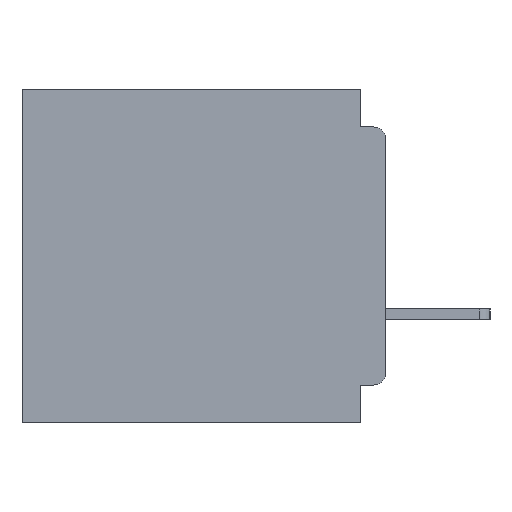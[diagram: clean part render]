
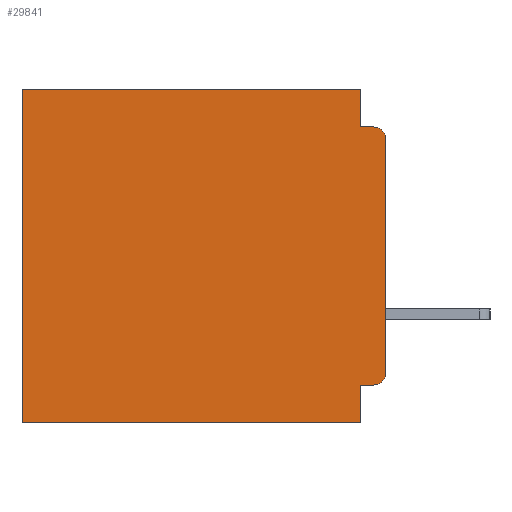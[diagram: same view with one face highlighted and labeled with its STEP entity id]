
A CAD part, left-side view. The second image highlights one B-rep face of the part: STEP entity #29841.
In plain terms, the highlighted planar face has unit normal (-1, 0, 0).
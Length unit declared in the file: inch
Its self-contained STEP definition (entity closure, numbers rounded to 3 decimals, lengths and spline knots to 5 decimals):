
#265 = VECTOR ( 'NONE', #46456, 39.37008 ) ;
#1572 = CARTESIAN_POINT ( 'NONE',  ( 0.3, 0.437, -0.4 ) ) ;
#1615 = EDGE_CURVE ( 'NONE', #7295, #20753, #33147, .T. ) ;
#2428 = LINE ( 'NONE', #33647, #3694 ) ;
#3460 = DIRECTION ( 'NONE',  ( 0., 1., 0. ) ) ;
#3662 = ORIENTED_EDGE ( 'NONE', *, *, #21971, .F. ) ;
#3694 = VECTOR ( 'NONE', #29589, 39.37008 ) ;
#4577 = DIRECTION ( 'NONE',  ( 1., 0., 0. ) ) ;
#5050 = VECTOR ( 'NONE', #21199, 39.37008 ) ;
#5406 = ORIENTED_EDGE ( 'NONE', *, *, #15258, .F. ) ;
#6187 = CARTESIAN_POINT ( 'NONE',  ( 0.3, 0.437, -0.4 ) ) ;
#6273 = ORIENTED_EDGE ( 'NONE', *, *, #46538, .F. ) ;
#6849 = EDGE_LOOP ( 'NONE', ( #51525, #38840, #45216, #6273, #16762, #49457, #3662, #35988, #5406, #42361 ) ) ;
#7295 = VERTEX_POINT ( 'NONE', #41009 ) ;
#7909 = DIRECTION ( 'NONE',  ( 0., 0., -1. ) ) ;
#9643 = VERTEX_POINT ( 'NONE', #45570 ) ;
#10082 = FACE_OUTER_BOUND ( 'NONE', #6849, .T. ) ;
#11104 = LINE ( 'NONE', #22349, #265 ) ;
#12404 = DIRECTION ( 'NONE',  ( 0., 0., -1. ) ) ;
#12607 = VECTOR ( 'NONE', #42141, 39.37008 ) ;
#12839 = VERTEX_POINT ( 'NONE', #47548 ) ;
#12994 = DIRECTION ( 'NONE',  ( -1., 0., 0. ) ) ;
#13832 = CARTESIAN_POINT ( 'NONE',  ( 0.3, 0., -0.4 ) ) ;
#13979 = VECTOR ( 'NONE', #3460, 39.37008 ) ;
#14029 = CARTESIAN_POINT ( 'NONE',  ( 0.3, 0., -0.34 ) ) ;
#15181 = LINE ( 'NONE', #13832, #12607 ) ;
#15258 = EDGE_CURVE ( 'NONE', #12839, #15596, #26531, .T. ) ;
#15596 = VERTEX_POINT ( 'NONE', #51578 ) ;
#16175 = CARTESIAN_POINT ( 'NONE',  ( 0.3, 0.031, -0.4 ) ) ;
#16762 = ORIENTED_EDGE ( 'NONE', *, *, #36141, .T. ) ;
#17529 = VECTOR ( 'NONE', #33875, 39.37008 ) ;
#17817 = CARTESIAN_POINT ( 'NONE',  ( 0.3, 0.015, -0.045 ) ) ;
#18796 = LINE ( 'NONE', #1572, #17529 ) ;
#19646 = EDGE_CURVE ( 'NONE', #7295, #28310, #43110, .T. ) ;
#20168 = VERTEX_POINT ( 'NONE', #46203 ) ;
#20345 = DIRECTION ( 'NONE',  ( -1., 0., 0. ) ) ;
#20721 = PLANE ( 'NONE',  #50280 ) ;
#20753 = VERTEX_POINT ( 'NONE', #17817 ) ;
#21199 = DIRECTION ( 'NONE',  ( 0., 1., 0. ) ) ;
#21971 = EDGE_CURVE ( 'NONE', #9643, #38137, #15181, .T. ) ;
#22255 = CARTESIAN_POINT ( 'NONE',  ( 0.3, 0.031, -0.045 ) ) ;
#22349 = CARTESIAN_POINT ( 'NONE',  ( 0.3, 0.031, 0. ) ) ;
#24540 = CARTESIAN_POINT ( 'NONE',  ( 0.3, 0., -0.4 ) ) ;
#26531 = LINE ( 'NONE', #49341, #5050 ) ;
#27902 = DIRECTION ( 'NONE',  ( 0., 0., -1. ) ) ;
#28310 = VERTEX_POINT ( 'NONE', #14029 ) ;
#28698 = CARTESIAN_POINT ( 'NONE',  ( 0.3, 0.015, -0.06 ) ) ;
#29589 = DIRECTION ( 'NONE',  ( 0., -1., 0. ) ) ;
#29841 = ADVANCED_FACE ( 'NONE', ( #10082 ), #20721, .F. ) ;
#29966 = AXIS2_PLACEMENT_3D ( 'NONE', #28698, #12994, #7909 ) ;
#32352 = VECTOR ( 'NONE', #12404, 39.37008 ) ;
#32781 = DIRECTION ( 'NONE',  ( 0., 0., -1. ) ) ;
#32958 = EDGE_CURVE ( 'NONE', #15596, #9643, #45087, .T. ) ;
#33018 = AXIS2_PLACEMENT_3D ( 'NONE', #44422, #20345, #48496 ) ;
#33069 = VECTOR ( 'NONE', #27902, 39.37008 ) ;
#33147 = CIRCLE ( 'NONE', #29966, 0.015 ) ;
#33647 = CARTESIAN_POINT ( 'NONE',  ( 0.3, 0., -0.045 ) ) ;
#33875 = DIRECTION ( 'NONE',  ( 0., 0., -1. ) ) ;
#34208 = VERTEX_POINT ( 'NONE', #22255 ) ;
#35339 = LINE ( 'NONE', #47908, #13979 ) ;
#35988 = ORIENTED_EDGE ( 'NONE', *, *, #32958, .F. ) ;
#36141 = EDGE_CURVE ( 'NONE', #20168, #50743, #35339, .T. ) ;
#36712 = CIRCLE ( 'NONE', #33018, 0.015 ) ;
#36767 = EDGE_CURVE ( 'NONE', #34208, #20753, #2428, .T. ) ;
#38037 = EDGE_CURVE ( 'NONE', #50743, #38137, #18796, .T. ) ;
#38137 = VERTEX_POINT ( 'NONE', #6187 ) ;
#38840 = ORIENTED_EDGE ( 'NONE', *, *, #1615, .T. ) ;
#39457 = CARTESIAN_POINT ( 'NONE',  ( 0.3, 0.437, 0. ) ) ;
#40481 = EDGE_CURVE ( 'NONE', #12839, #28310, #36712, .T. ) ;
#41009 = CARTESIAN_POINT ( 'NONE',  ( 0.3, 0., -0.06 ) ) ;
#42141 = DIRECTION ( 'NONE',  ( 0., 1., 0. ) ) ;
#42361 = ORIENTED_EDGE ( 'NONE', *, *, #40481, .T. ) ;
#43110 = LINE ( 'NONE', #24540, #32352 ) ;
#44422 = CARTESIAN_POINT ( 'NONE',  ( 0.3, 0.015, -0.34 ) ) ;
#44820 = CARTESIAN_POINT ( 'NONE',  ( 0.3, 0., -0.4 ) ) ;
#45087 = LINE ( 'NONE', #16175, #33069 ) ;
#45216 = ORIENTED_EDGE ( 'NONE', *, *, #36767, .F. ) ;
#45570 = CARTESIAN_POINT ( 'NONE',  ( 0.3, 0.031, -0.4 ) ) ;
#46203 = CARTESIAN_POINT ( 'NONE',  ( 0.3, 0.031, 0. ) ) ;
#46456 = DIRECTION ( 'NONE',  ( 0., 0., -1. ) ) ;
#46538 = EDGE_CURVE ( 'NONE', #20168, #34208, #11104, .T. ) ;
#47548 = CARTESIAN_POINT ( 'NONE',  ( 0.3, 0.015, -0.355 ) ) ;
#47908 = CARTESIAN_POINT ( 'NONE',  ( 0.3, 0., 0. ) ) ;
#48496 = DIRECTION ( 'NONE',  ( 0., 0., -1. ) ) ;
#49341 = CARTESIAN_POINT ( 'NONE',  ( 0.3, 0., -0.355 ) ) ;
#49457 = ORIENTED_EDGE ( 'NONE', *, *, #38037, .T. ) ;
#50280 = AXIS2_PLACEMENT_3D ( 'NONE', #44820, #4577, #32781 ) ;
#50743 = VERTEX_POINT ( 'NONE', #39457 ) ;
#51525 = ORIENTED_EDGE ( 'NONE', *, *, #19646, .F. ) ;
#51578 = CARTESIAN_POINT ( 'NONE',  ( 0.3, 0.031, -0.355 ) ) ;
